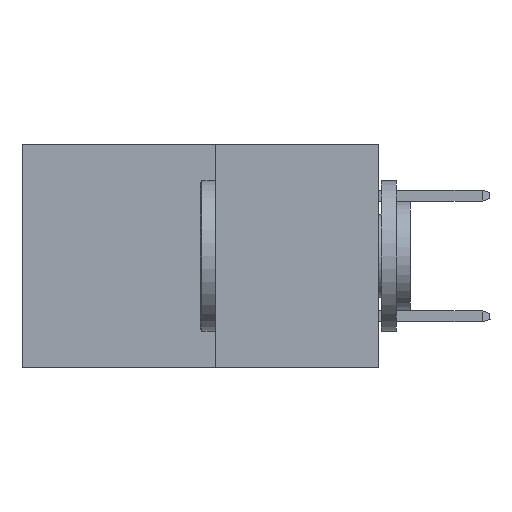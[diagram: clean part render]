
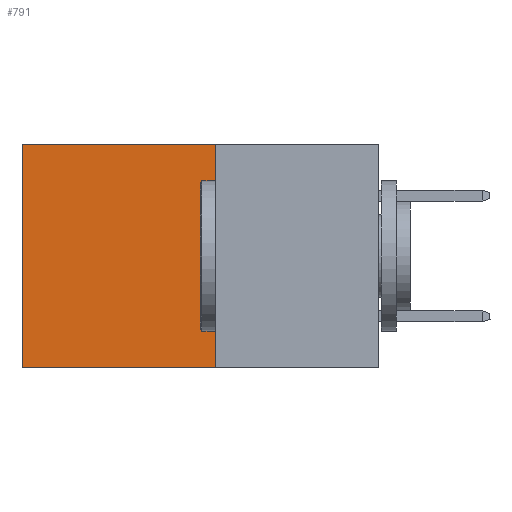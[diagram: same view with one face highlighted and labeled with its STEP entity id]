
A CAD part, left-side view. The second image highlights one B-rep face of the part: STEP entity #791.
In plain terms, the highlighted planar face has unit normal (-1, 0, 0).
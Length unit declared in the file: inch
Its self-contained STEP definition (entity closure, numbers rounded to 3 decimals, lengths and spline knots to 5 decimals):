
#791 = ADVANCED_FACE ( 'NONE', ( #20655 ), #14472, .F. ) ;
#1635 = ORIENTED_EDGE ( 'NONE', *, *, #6930, .T. ) ;
#2233 = EDGE_CURVE ( 'NONE', #11669, #6568, #10108, .T. ) ;
#2698 = CARTESIAN_POINT ( 'NONE',  ( 0.277, 0.27, -0.37 ) ) ;
#3305 = CARTESIAN_POINT ( 'NONE',  ( 0.277, 0.27, 0. ) ) ;
#4875 = CARTESIAN_POINT ( 'NONE',  ( 0.277, 0.27, -0.37 ) ) ;
#5547 = DIRECTION ( 'NONE',  ( 0., 0., -1. ) ) ;
#6046 = EDGE_LOOP ( 'NONE', ( #8222, #8205, #17474, #1635 ) ) ;
#6568 = VERTEX_POINT ( 'NONE', #10582 ) ;
#6642 = VECTOR ( 'NONE', #17823, 39.37008 ) ;
#6930 = EDGE_CURVE ( 'NONE', #20505, #11669, #6953, .T. ) ;
#6953 = LINE ( 'NONE', #11472, #21706 ) ;
#7556 = CARTESIAN_POINT ( 'NONE',  ( 0.277, 0.27, -0.37 ) ) ;
#8205 = ORIENTED_EDGE ( 'NONE', *, *, #16784, .F. ) ;
#8222 = ORIENTED_EDGE ( 'NONE', *, *, #2233, .T. ) ;
#9417 = DIRECTION ( 'NONE',  ( 0., 0., -1. ) ) ;
#9832 = DIRECTION ( 'NONE',  ( 0., 0., -1. ) ) ;
#9900 = CARTESIAN_POINT ( 'NONE',  ( 0.277, 0.59, -0.37 ) ) ;
#10108 = LINE ( 'NONE', #9900, #15060 ) ;
#10582 = CARTESIAN_POINT ( 'NONE',  ( 0.277, 0.59, -0.37 ) ) ;
#11472 = CARTESIAN_POINT ( 'NONE',  ( 0.277, 0.27, 0. ) ) ;
#11669 = VERTEX_POINT ( 'NONE', #22025 ) ;
#12236 = LINE ( 'NONE', #7556, #16018 ) ;
#12547 = AXIS2_PLACEMENT_3D ( 'NONE', #14443, #20766, #9832 ) ;
#13322 = DIRECTION ( 'NONE',  ( 0., 1., 0. ) ) ;
#13811 = EDGE_CURVE ( 'NONE', #20505, #16205, #12236, .T. ) ;
#14443 = CARTESIAN_POINT ( 'NONE',  ( 0.277, 0.27, -0.37 ) ) ;
#14472 = PLANE ( 'NONE',  #12547 ) ;
#15060 = VECTOR ( 'NONE', #5547, 39.37008 ) ;
#15332 = LINE ( 'NONE', #4875, #6642 ) ;
#16018 = VECTOR ( 'NONE', #9417, 39.37008 ) ;
#16205 = VERTEX_POINT ( 'NONE', #2698 ) ;
#16784 = EDGE_CURVE ( 'NONE', #16205, #6568, #15332, .T. ) ;
#17474 = ORIENTED_EDGE ( 'NONE', *, *, #13811, .F. ) ;
#17823 = DIRECTION ( 'NONE',  ( 0., 1., 0. ) ) ;
#20505 = VERTEX_POINT ( 'NONE', #3305 ) ;
#20655 = FACE_OUTER_BOUND ( 'NONE', #6046, .T. ) ;
#20766 = DIRECTION ( 'NONE',  ( 1., 0., 0. ) ) ;
#21706 = VECTOR ( 'NONE', #13322, 39.37008 ) ;
#22025 = CARTESIAN_POINT ( 'NONE',  ( 0.277, 0.59, 0. ) ) ;
